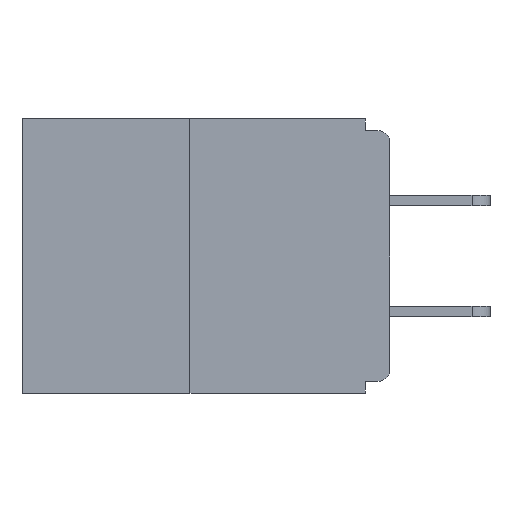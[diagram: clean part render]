
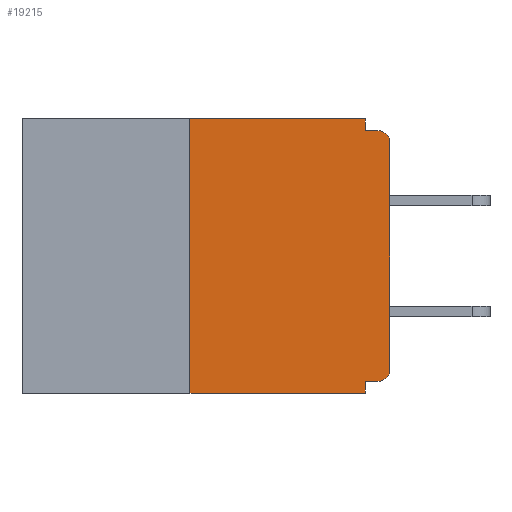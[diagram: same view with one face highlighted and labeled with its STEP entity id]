
A CAD part, left-side view. The second image highlights one B-rep face of the part: STEP entity #19215.
In plain terms, the highlighted planar face has unit normal (-1, 0, 0).
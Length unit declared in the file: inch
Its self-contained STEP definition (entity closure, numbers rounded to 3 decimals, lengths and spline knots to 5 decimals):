
#556 = EDGE_CURVE ( 'NONE', #11615, #3145, #23748, .T. ) ;
#773 = VERTEX_POINT ( 'NONE', #18563 ) ;
#2532 = PLANE ( 'NONE',  #30997 ) ;
#2864 = DIRECTION ( 'NONE',  ( 0., 0., -1. ) ) ;
#3083 = ORIENTED_EDGE ( 'NONE', *, *, #7516, .F. ) ;
#3145 = VERTEX_POINT ( 'NONE', #26312 ) ;
#3380 = VECTOR ( 'NONE', #26202, 39.37008 ) ;
#3452 = LINE ( 'NONE', #30636, #23393 ) ;
#3574 = ORIENTED_EDGE ( 'NONE', *, *, #13955, .F. ) ;
#5172 = CARTESIAN_POINT ( 'NONE',  ( 0., 0., -0.015 ) ) ;
#6740 = LINE ( 'NONE', #23804, #3380 ) ;
#6859 = CIRCLE ( 'NONE', #11051, 0.015 ) ;
#7238 = DIRECTION ( 'NONE',  ( 1., 0., 0. ) ) ;
#7516 = EDGE_CURVE ( 'NONE', #14457, #23172, #29885, .T. ) ;
#7594 = EDGE_CURVE ( 'NONE', #30875, #14457, #12174, .T. ) ;
#7884 = CARTESIAN_POINT ( 'NONE',  ( 0., 0.031, 0. ) ) ;
#7938 = FACE_OUTER_BOUND ( 'NONE', #18808, .T. ) ;
#8084 = DIRECTION ( 'NONE',  ( 0., 0., -1. ) ) ;
#8372 = CARTESIAN_POINT ( 'NONE',  ( 0., 0.015, -0.313 ) ) ;
#8573 = DIRECTION ( 'NONE',  ( 0., 0., -1. ) ) ;
#9556 = VERTEX_POINT ( 'NONE', #27963 ) ;
#10154 = DIRECTION ( 'NONE',  ( 0., -1., 0. ) ) ;
#10362 = CARTESIAN_POINT ( 'NONE',  ( 0., 0., -0.313 ) ) ;
#10873 = ORIENTED_EDGE ( 'NONE', *, *, #7594, .F. ) ;
#11051 = AXIS2_PLACEMENT_3D ( 'NONE', #8372, #22680, #8573 ) ;
#11097 = ORIENTED_EDGE ( 'NONE', *, *, #19531, .T. ) ;
#11509 = ORIENTED_EDGE ( 'NONE', *, *, #556, .T. ) ;
#11615 = VERTEX_POINT ( 'NONE', #13328 ) ;
#12174 = LINE ( 'NONE', #7884, #16684 ) ;
#13328 = CARTESIAN_POINT ( 'NONE',  ( 0., 0.25, -0.343 ) ) ;
#13338 = CARTESIAN_POINT ( 'NONE',  ( 0., 0.015, -0.03 ) ) ;
#13955 = EDGE_CURVE ( 'NONE', #9556, #3145, #3452, .T. ) ;
#14457 = VERTEX_POINT ( 'NONE', #19505 ) ;
#16684 = VECTOR ( 'NONE', #2864, 39.37008 ) ;
#16915 = CARTESIAN_POINT ( 'NONE',  ( 0., 0.46, 0. ) ) ;
#17015 = DIRECTION ( 'NONE',  ( 0., 0., -1. ) ) ;
#18188 = ORIENTED_EDGE ( 'NONE', *, *, #18819, .T. ) ;
#18219 = VERTEX_POINT ( 'NONE', #26970 ) ;
#18563 = CARTESIAN_POINT ( 'NONE',  ( 0., 0., -0.03 ) ) ;
#18631 = DIRECTION ( 'NONE',  ( 0., 0., -1. ) ) ;
#18808 = EDGE_LOOP ( 'NONE', ( #26593, #20745, #11509, #3574, #29751, #18188, #23796, #11097, #3083, #10873 ) ) ;
#18819 = EDGE_CURVE ( 'NONE', #25665, #22533, #6859, .T. ) ;
#19215 = ADVANCED_FACE ( 'NONE', ( #7938 ), #2532, .F. ) ;
#19505 = CARTESIAN_POINT ( 'NONE',  ( 0., 0.031, -0.015 ) ) ;
#19531 = EDGE_CURVE ( 'NONE', #773, #23172, #26339, .T. ) ;
#20332 = CARTESIAN_POINT ( 'NONE',  ( 0., 0.031, 0. ) ) ;
#20413 = EDGE_CURVE ( 'NONE', #22533, #773, #30374, .T. ) ;
#20745 = ORIENTED_EDGE ( 'NONE', *, *, #24827, .F. ) ;
#20872 = VECTOR ( 'NONE', #27139, 39.37008 ) ;
#21473 = VECTOR ( 'NONE', #10154, 39.37008 ) ;
#21875 = CARTESIAN_POINT ( 'NONE',  ( 0., 0., 0. ) ) ;
#22075 = LINE ( 'NONE', #27559, #26955 ) ;
#22504 = DIRECTION ( 'NONE',  ( -1., 0., 0. ) ) ;
#22533 = VERTEX_POINT ( 'NONE', #10362 ) ;
#22680 = DIRECTION ( 'NONE',  ( -1., 0., 0. ) ) ;
#23030 = CARTESIAN_POINT ( 'NONE',  ( 0., 0.015, -0.015 ) ) ;
#23172 = VERTEX_POINT ( 'NONE', #23030 ) ;
#23393 = VECTOR ( 'NONE', #18631, 39.37008 ) ;
#23748 = LINE ( 'NONE', #26776, #21473 ) ;
#23796 = ORIENTED_EDGE ( 'NONE', *, *, #20413, .T. ) ;
#23804 = CARTESIAN_POINT ( 'NONE',  ( 0., 0.46, 0. ) ) ;
#24827 = EDGE_CURVE ( 'NONE', #11615, #18219, #22075, .T. ) ;
#25301 = DIRECTION ( 'NONE',  ( 0., 1., 0. ) ) ;
#25665 = VERTEX_POINT ( 'NONE', #26956 ) ;
#26202 = DIRECTION ( 'NONE',  ( 0., -1., 0. ) ) ;
#26312 = CARTESIAN_POINT ( 'NONE',  ( 0., 0.031, -0.343 ) ) ;
#26339 = CIRCLE ( 'NONE', #30814, 0.015 ) ;
#26593 = ORIENTED_EDGE ( 'NONE', *, *, #27923, .F. ) ;
#26776 = CARTESIAN_POINT ( 'NONE',  ( 0., 0.46, -0.343 ) ) ;
#26781 = DIRECTION ( 'NONE',  ( 0., 0., 1. ) ) ;
#26901 = DIRECTION ( 'NONE',  ( 0., 0., 1. ) ) ;
#26913 = VECTOR ( 'NONE', #26901, 39.37008 ) ;
#26955 = VECTOR ( 'NONE', #26781, 39.37008 ) ;
#26956 = CARTESIAN_POINT ( 'NONE',  ( 0., 0.015, -0.328 ) ) ;
#26970 = CARTESIAN_POINT ( 'NONE',  ( 0., 0.25, 0. ) ) ;
#27101 = LINE ( 'NONE', #30241, #30888 ) ;
#27139 = DIRECTION ( 'NONE',  ( 0., -1., 0. ) ) ;
#27191 = EDGE_CURVE ( 'NONE', #25665, #9556, #27101, .T. ) ;
#27559 = CARTESIAN_POINT ( 'NONE',  ( 0., 0.25, 0. ) ) ;
#27923 = EDGE_CURVE ( 'NONE', #18219, #30875, #6740, .T. ) ;
#27963 = CARTESIAN_POINT ( 'NONE',  ( 0., 0.031, -0.328 ) ) ;
#29751 = ORIENTED_EDGE ( 'NONE', *, *, #27191, .F. ) ;
#29885 = LINE ( 'NONE', #5172, #20872 ) ;
#30241 = CARTESIAN_POINT ( 'NONE',  ( 0., 0., -0.328 ) ) ;
#30374 = LINE ( 'NONE', #21875, #26913 ) ;
#30636 = CARTESIAN_POINT ( 'NONE',  ( 0., 0.031, -0.343 ) ) ;
#30814 = AXIS2_PLACEMENT_3D ( 'NONE', #13338, #22504, #8084 ) ;
#30875 = VERTEX_POINT ( 'NONE', #20332 ) ;
#30888 = VECTOR ( 'NONE', #25301, 39.37008 ) ;
#30997 = AXIS2_PLACEMENT_3D ( 'NONE', #16915, #7238, #17015 ) ;
